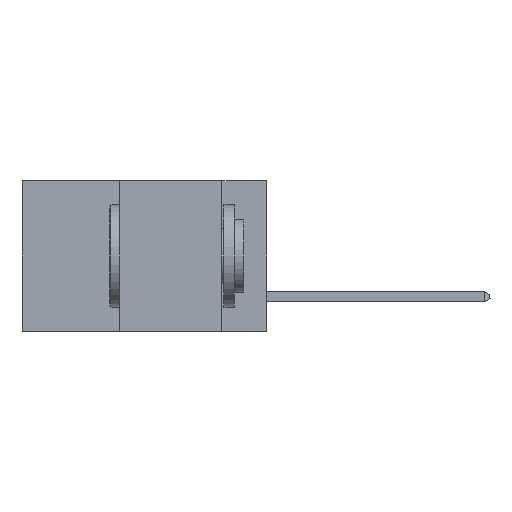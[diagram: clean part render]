
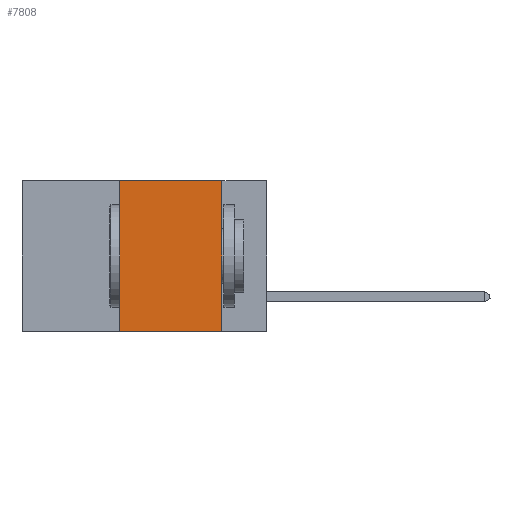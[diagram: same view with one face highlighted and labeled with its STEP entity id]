
A CAD part, left-side view. The second image highlights one B-rep face of the part: STEP entity #7808.
In plain terms, the highlighted planar face has unit normal (-1, 0, 0).
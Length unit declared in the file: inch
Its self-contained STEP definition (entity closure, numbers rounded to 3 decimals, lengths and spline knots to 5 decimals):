
#625 = CARTESIAN_POINT ( 'NONE',  ( 0., 0.6, 0. ) ) ;
#1218 = ORIENTED_EDGE ( 'NONE', *, *, #20595, .T. ) ;
#2931 = VERTEX_POINT ( 'NONE', #3064 ) ;
#3064 = CARTESIAN_POINT ( 'NONE',  ( 0., 0.11, 0. ) ) ;
#3480 = CARTESIAN_POINT ( 'NONE',  ( 0., 0.36, 0. ) ) ;
#3880 = LINE ( 'NONE', #18517, #15079 ) ;
#5288 = ORIENTED_EDGE ( 'NONE', *, *, #14003, .F. ) ;
#5711 = DIRECTION ( 'NONE',  ( 0., -1., 0. ) ) ;
#5906 = FACE_OUTER_BOUND ( 'NONE', #12934, .T. ) ;
#6641 = LINE ( 'NONE', #13371, #10336 ) ;
#7503 = DIRECTION ( 'NONE',  ( 0., 0., 1. ) ) ;
#7511 = CARTESIAN_POINT ( 'NONE',  ( 0., 0.6, -0.37 ) ) ;
#7808 = ADVANCED_FACE ( 'NONE', ( #5906 ), #18116, .F. ) ;
#7871 = EDGE_CURVE ( 'NONE', #2931, #18556, #6641, .T. ) ;
#8322 = DIRECTION ( 'NONE',  ( 0., 0., -1. ) ) ;
#8484 = EDGE_CURVE ( 'NONE', #13099, #13376, #14829, .T. ) ;
#8659 = ORIENTED_EDGE ( 'NONE', *, *, #8484, .F. ) ;
#8946 = CARTESIAN_POINT ( 'NONE',  ( 0., 0.36, 0. ) ) ;
#9093 = VECTOR ( 'NONE', #7503, 39.37008 ) ;
#10336 = VECTOR ( 'NONE', #18660, 39.37008 ) ;
#12532 = AXIS2_PLACEMENT_3D ( 'NONE', #625, #13036, #8322 ) ;
#12934 = EDGE_LOOP ( 'NONE', ( #15441, #5288, #8659, #1218 ) ) ;
#13036 = DIRECTION ( 'NONE',  ( 1., 0., 0. ) ) ;
#13099 = VERTEX_POINT ( 'NONE', #18827 ) ;
#13371 = CARTESIAN_POINT ( 'NONE',  ( 0., 0.11, 0. ) ) ;
#13376 = VERTEX_POINT ( 'NONE', #3480 ) ;
#14003 = EDGE_CURVE ( 'NONE', #13376, #2931, #3880, .T. ) ;
#14829 = LINE ( 'NONE', #8946, #9093 ) ;
#15079 = VECTOR ( 'NONE', #5711, 39.37008 ) ;
#15441 = ORIENTED_EDGE ( 'NONE', *, *, #7871, .F. ) ;
#17211 = CARTESIAN_POINT ( 'NONE',  ( 0., 0.11, -0.37 ) ) ;
#17907 = LINE ( 'NONE', #7511, #20145 ) ;
#18116 = PLANE ( 'NONE',  #12532 ) ;
#18517 = CARTESIAN_POINT ( 'NONE',  ( 0., 0.6, 0. ) ) ;
#18556 = VERTEX_POINT ( 'NONE', #17211 ) ;
#18660 = DIRECTION ( 'NONE',  ( 0., 0., -1. ) ) ;
#18697 = DIRECTION ( 'NONE',  ( 0., -1., 0. ) ) ;
#18827 = CARTESIAN_POINT ( 'NONE',  ( 0., 0.36, -0.37 ) ) ;
#20145 = VECTOR ( 'NONE', #18697, 39.37008 ) ;
#20595 = EDGE_CURVE ( 'NONE', #13099, #18556, #17907, .T. ) ;
